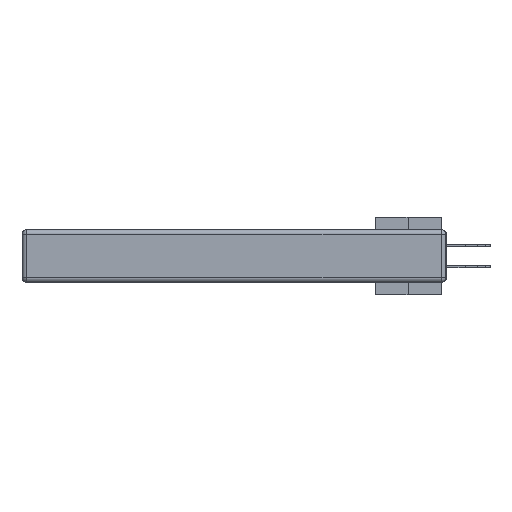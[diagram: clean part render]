
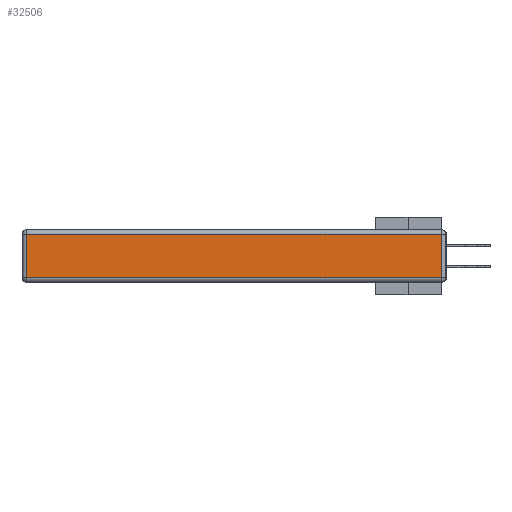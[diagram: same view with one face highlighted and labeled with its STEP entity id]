
A CAD part, left-side view. The second image highlights one B-rep face of the part: STEP entity #32506.
In plain terms, the highlighted planar face has unit normal (-1, 0, 0).
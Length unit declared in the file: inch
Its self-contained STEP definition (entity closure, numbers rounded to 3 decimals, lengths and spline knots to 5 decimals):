
#1229 = EDGE_CURVE ( 'NONE', #7090, #30985, #2237, .T. ) ;
#2237 = LINE ( 'NONE', #8386, #31434 ) ;
#3151 = ORIENTED_EDGE ( 'NONE', *, *, #38481, .T. ) ;
#4392 = VERTEX_POINT ( 'NONE', #36305 ) ;
#4534 = DIRECTION ( 'NONE',  ( 0., 0., -1. ) ) ;
#6316 = CARTESIAN_POINT ( 'NONE',  ( 0., 0.03, -0.313 ) ) ;
#6959 = FACE_OUTER_BOUND ( 'NONE', #25456, .T. ) ;
#7090 = VERTEX_POINT ( 'NONE', #6316 ) ;
#7817 = VERTEX_POINT ( 'NONE', #35368 ) ;
#8054 = VECTOR ( 'NONE', #11459, 39.37008 ) ;
#8386 = CARTESIAN_POINT ( 'NONE',  ( 0., 0.03, -0.343 ) ) ;
#11427 = PLANE ( 'NONE',  #38233 ) ;
#11459 = DIRECTION ( 'NONE',  ( 0., -1., 0. ) ) ;
#11546 = LINE ( 'NONE', #34452, #26814 ) ;
#11739 = LINE ( 'NONE', #12702, #31781 ) ;
#12702 = CARTESIAN_POINT ( 'NONE',  ( 0., 2.75, -0.03 ) ) ;
#14939 = ORIENTED_EDGE ( 'NONE', *, *, #30149, .T. ) ;
#18674 = CARTESIAN_POINT ( 'NONE',  ( 0., 0.03, -0.03 ) ) ;
#19067 = CARTESIAN_POINT ( 'NONE',  ( 0., 0., -0.313 ) ) ;
#23165 = ORIENTED_EDGE ( 'NONE', *, *, #23296, .T. ) ;
#23296 = EDGE_CURVE ( 'NONE', #30985, #7817, #11739, .T. ) ;
#25456 = EDGE_LOOP ( 'NONE', ( #14939, #39104, #23165, #3151 ) ) ;
#26814 = VECTOR ( 'NONE', #4534, 39.37008 ) ;
#26899 = DIRECTION ( 'NONE',  ( -1., 0., 0. ) ) ;
#27647 = LINE ( 'NONE', #19067, #8054 ) ;
#30149 = EDGE_CURVE ( 'NONE', #4392, #7090, #27647, .T. ) ;
#30985 = VERTEX_POINT ( 'NONE', #18674 ) ;
#31434 = VECTOR ( 'NONE', #38959, 39.37008 ) ;
#31781 = VECTOR ( 'NONE', #33528, 39.37008 ) ;
#32506 = ADVANCED_FACE ( 'NONE', ( #6959 ), #11427, .T. ) ;
#33174 = CARTESIAN_POINT ( 'NONE',  ( 0., 0., -0.343 ) ) ;
#33528 = DIRECTION ( 'NONE',  ( 0., 1., 0. ) ) ;
#34452 = CARTESIAN_POINT ( 'NONE',  ( 0., 2.72, -0.343 ) ) ;
#35368 = CARTESIAN_POINT ( 'NONE',  ( 0., 2.72, -0.03 ) ) ;
#35823 = DIRECTION ( 'NONE',  ( 0., 0., 1. ) ) ;
#36305 = CARTESIAN_POINT ( 'NONE',  ( 0., 2.72, -0.313 ) ) ;
#38233 = AXIS2_PLACEMENT_3D ( 'NONE', #33174, #26899, #35823 ) ;
#38481 = EDGE_CURVE ( 'NONE', #7817, #4392, #11546, .T. ) ;
#38959 = DIRECTION ( 'NONE',  ( 0., 0., 1. ) ) ;
#39104 = ORIENTED_EDGE ( 'NONE', *, *, #1229, .T. ) ;
